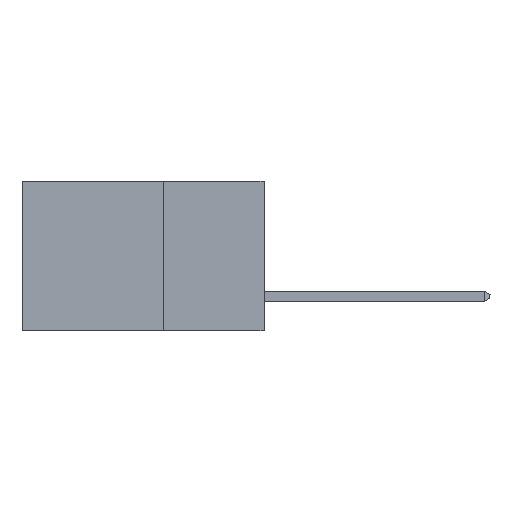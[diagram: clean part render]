
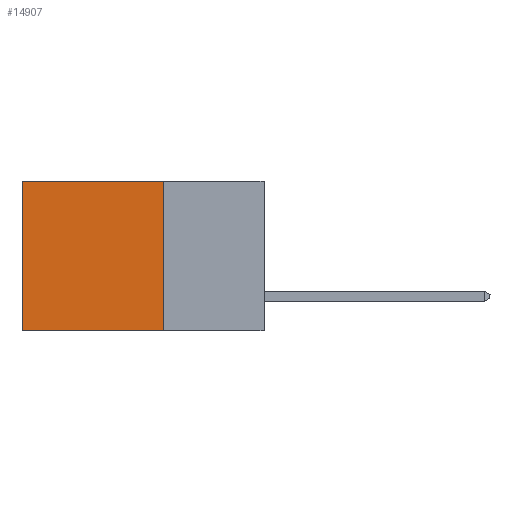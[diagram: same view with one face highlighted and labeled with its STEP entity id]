
A CAD part, left-side view. The second image highlights one B-rep face of the part: STEP entity #14907.
In plain terms, the highlighted planar face has unit normal (-1, 0, 0).
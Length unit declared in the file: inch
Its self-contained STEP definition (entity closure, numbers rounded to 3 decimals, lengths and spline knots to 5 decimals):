
#189 = FACE_OUTER_BOUND ( 'NONE', #10165, .T. ) ;
#223 = VERTEX_POINT ( 'NONE', #10188 ) ;
#689 = CARTESIAN_POINT ( 'NONE',  ( 0.2615, 0.25, -0.37 ) ) ;
#1578 = LINE ( 'NONE', #8799, #11164 ) ;
#1676 = VERTEX_POINT ( 'NONE', #5949 ) ;
#1903 = CARTESIAN_POINT ( 'NONE',  ( 0.2615, 0.6, -0.37 ) ) ;
#2118 = VERTEX_POINT ( 'NONE', #7563 ) ;
#2877 = LINE ( 'NONE', #17737, #15419 ) ;
#4155 = EDGE_CURVE ( 'NONE', #2118, #223, #2877, .T. ) ;
#4424 = CARTESIAN_POINT ( 'NONE',  ( 0.2615, 0.25, -0.37 ) ) ;
#4544 = CARTESIAN_POINT ( 'NONE',  ( 0.2615, 0.25, -0.37 ) ) ;
#5186 = EDGE_CURVE ( 'NONE', #16220, #1676, #1578, .T. ) ;
#5675 = DIRECTION ( 'NONE',  ( 0., 0., -1. ) ) ;
#5949 = CARTESIAN_POINT ( 'NONE',  ( 0.2615, 0.6, -0.37 ) ) ;
#7402 = PLANE ( 'NONE',  #16399 ) ;
#7563 = CARTESIAN_POINT ( 'NONE',  ( 0.2615, 0.25, 0. ) ) ;
#8743 = DIRECTION ( 'NONE',  ( 0., 1., 0. ) ) ;
#8799 = CARTESIAN_POINT ( 'NONE',  ( 0.2615, 0.25, -0.37 ) ) ;
#8834 = VECTOR ( 'NONE', #13761, 39.37008 ) ;
#9014 = LINE ( 'NONE', #1903, #17721 ) ;
#10165 = EDGE_LOOP ( 'NONE', ( #13354, #13255, #17161, #15112 ) ) ;
#10188 = CARTESIAN_POINT ( 'NONE',  ( 0.2615, 0.6, 0. ) ) ;
#10696 = EDGE_CURVE ( 'NONE', #223, #1676, #9014, .T. ) ;
#11164 = VECTOR ( 'NONE', #14646, 39.37008 ) ;
#13255 = ORIENTED_EDGE ( 'NONE', *, *, #5186, .F. ) ;
#13354 = ORIENTED_EDGE ( 'NONE', *, *, #10696, .T. ) ;
#13761 = DIRECTION ( 'NONE',  ( 0., 0., -1. ) ) ;
#14505 = DIRECTION ( 'NONE',  ( 1., 0., 0. ) ) ;
#14646 = DIRECTION ( 'NONE',  ( 0., 1., 0. ) ) ;
#14768 = DIRECTION ( 'NONE',  ( 0., 0., -1. ) ) ;
#14907 = ADVANCED_FACE ( 'NONE', ( #189 ), #7402, .F. ) ;
#15112 = ORIENTED_EDGE ( 'NONE', *, *, #4155, .T. ) ;
#15419 = VECTOR ( 'NONE', #8743, 39.37008 ) ;
#16220 = VERTEX_POINT ( 'NONE', #4544 ) ;
#16399 = AXIS2_PLACEMENT_3D ( 'NONE', #4424, #14505, #5675 ) ;
#17161 = ORIENTED_EDGE ( 'NONE', *, *, #17532, .F. ) ;
#17532 = EDGE_CURVE ( 'NONE', #2118, #16220, #17866, .T. ) ;
#17721 = VECTOR ( 'NONE', #14768, 39.37008 ) ;
#17737 = CARTESIAN_POINT ( 'NONE',  ( 0.2615, 0.25, 0. ) ) ;
#17866 = LINE ( 'NONE', #689, #8834 ) ;
